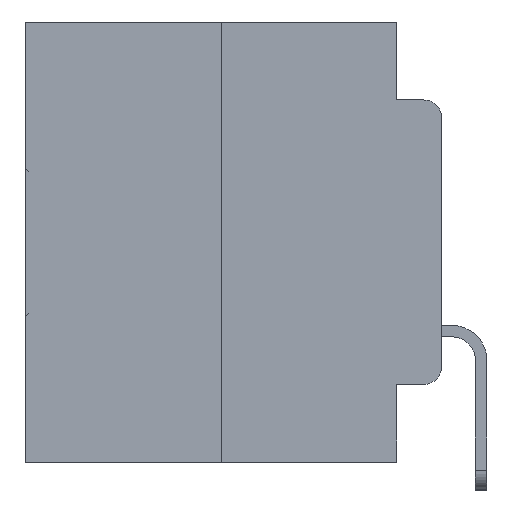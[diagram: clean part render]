
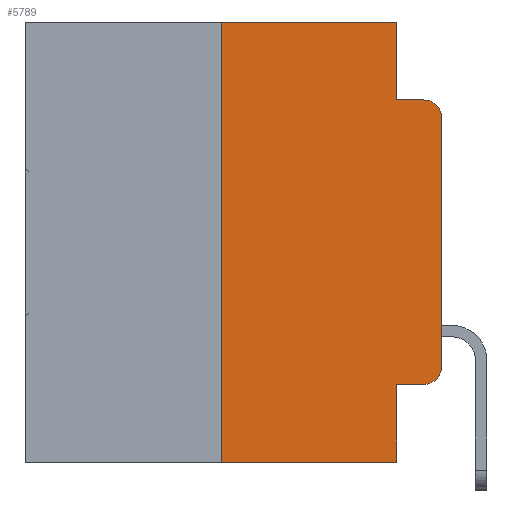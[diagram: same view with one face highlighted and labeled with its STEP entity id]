
A CAD part, left-side view. The second image highlights one B-rep face of the part: STEP entity #5789.
In plain terms, the highlighted planar face has unit normal (-1, 0, 0).
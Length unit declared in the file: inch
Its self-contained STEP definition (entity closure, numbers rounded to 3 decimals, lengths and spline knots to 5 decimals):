
#359 = VERTEX_POINT ( 'NONE', #4496 ) ;
#924 = VERTEX_POINT ( 'NONE', #22224 ) ;
#1751 = LINE ( 'NONE', #13528, #19166 ) ;
#1945 = LINE ( 'NONE', #23768, #21489 ) ;
#2202 = VERTEX_POINT ( 'NONE', #22669 ) ;
#2836 = CARTESIAN_POINT ( 'NONE',  ( 0., 0.051, 0. ) ) ;
#3096 = VERTEX_POINT ( 'NONE', #24365 ) ;
#3116 = PLANE ( 'NONE',  #24971 ) ;
#3329 = DIRECTION ( 'NONE',  ( 0., 0., -1. ) ) ;
#4472 = VECTOR ( 'NONE', #3329, 39.37008 ) ;
#4486 = CARTESIAN_POINT ( 'NONE',  ( 0., 0.02, -0.1085 ) ) ;
#4496 = CARTESIAN_POINT ( 'NONE',  ( 0., 0.051, -0.0885 ) ) ;
#4574 = DIRECTION ( 'NONE',  ( 0., 0., -1. ) ) ;
#4781 = CARTESIAN_POINT ( 'NONE',  ( 0., 0., 0. ) ) ;
#4948 = DIRECTION ( 'NONE',  ( -1., 0., 0. ) ) ;
#5156 = VERTEX_POINT ( 'NONE', #26609 ) ;
#5623 = CIRCLE ( 'NONE', #19106, 0.02 ) ;
#5789 = ADVANCED_FACE ( 'NONE', ( #25299 ), #3116, .F. ) ;
#6085 = LINE ( 'NONE', #24752, #14557 ) ;
#7357 = VECTOR ( 'NONE', #22712, 39.37008 ) ;
#7671 = EDGE_CURVE ( 'NONE', #359, #26872, #6085, .T. ) ;
#7709 = CARTESIAN_POINT ( 'NONE',  ( 0., 0.051, 0. ) ) ;
#7758 = LINE ( 'NONE', #12530, #8471 ) ;
#7809 = AXIS2_PLACEMENT_3D ( 'NONE', #18550, #4948, #20825 ) ;
#7986 = ORIENTED_EDGE ( 'NONE', *, *, #7671, .F. ) ;
#8322 = EDGE_CURVE ( 'NONE', #11139, #23448, #1751, .T. ) ;
#8471 = VECTOR ( 'NONE', #23954, 39.37008 ) ;
#8658 = EDGE_CURVE ( 'NONE', #20943, #26930, #7758, .T. ) ;
#8813 = DIRECTION ( 'NONE',  ( 0., -1., 0. ) ) ;
#9169 = EDGE_CURVE ( 'NONE', #20943, #11139, #15193, .T. ) ;
#10482 = EDGE_CURVE ( 'NONE', #3096, #924, #17296, .T. ) ;
#11045 = VECTOR ( 'NONE', #11236, 39.37008 ) ;
#11139 = VERTEX_POINT ( 'NONE', #11206 ) ;
#11167 = EDGE_CURVE ( 'NONE', #924, #26872, #5623, .T. ) ;
#11206 = CARTESIAN_POINT ( 'NONE',  ( 0., 0.25, 0. ) ) ;
#11236 = DIRECTION ( 'NONE',  ( 0., 0., -1. ) ) ;
#11402 = ORIENTED_EDGE ( 'NONE', *, *, #8322, .F. ) ;
#11656 = VECTOR ( 'NONE', #15746, 39.37008 ) ;
#12154 = ORIENTED_EDGE ( 'NONE', *, *, #26990, .T. ) ;
#12530 = CARTESIAN_POINT ( 'NONE',  ( 0., 0.473, -0.5 ) ) ;
#12810 = ORIENTED_EDGE ( 'NONE', *, *, #9169, .F. ) ;
#12998 = ORIENTED_EDGE ( 'NONE', *, *, #10482, .T. ) ;
#13528 = CARTESIAN_POINT ( 'NONE',  ( 0., 0.473, 0. ) ) ;
#14422 = CARTESIAN_POINT ( 'NONE',  ( 0., 0.051, -0.5 ) ) ;
#14557 = VECTOR ( 'NONE', #8813, 39.37008 ) ;
#14722 = CARTESIAN_POINT ( 'NONE',  ( 0., 0.02, -0.0885 ) ) ;
#15089 = DIRECTION ( 'NONE',  ( 0., 0., -1. ) ) ;
#15157 = EDGE_CURVE ( 'NONE', #5156, #26930, #21157, .T. ) ;
#15193 = LINE ( 'NONE', #27140, #11656 ) ;
#15746 = DIRECTION ( 'NONE',  ( 0., 0., 1. ) ) ;
#16046 = EDGE_CURVE ( 'NONE', #2202, #3096, #25396, .T. ) ;
#17296 = LINE ( 'NONE', #4781, #7357 ) ;
#17542 = ORIENTED_EDGE ( 'NONE', *, *, #22540, .F. ) ;
#18465 = DIRECTION ( 'NONE',  ( -1., 0., 0. ) ) ;
#18550 = CARTESIAN_POINT ( 'NONE',  ( 0., 0.02, -0.3915 ) ) ;
#18883 = ORIENTED_EDGE ( 'NONE', *, *, #16046, .T. ) ;
#19106 = AXIS2_PLACEMENT_3D ( 'NONE', #4486, #18465, #4574 ) ;
#19166 = VECTOR ( 'NONE', #20363, 39.37008 ) ;
#20363 = DIRECTION ( 'NONE',  ( 0., -1., 0. ) ) ;
#20825 = DIRECTION ( 'NONE',  ( 0., 0., -1. ) ) ;
#20943 = VERTEX_POINT ( 'NONE', #24436 ) ;
#21157 = LINE ( 'NONE', #2836, #4472 ) ;
#21489 = VECTOR ( 'NONE', #28393, 39.37008 ) ;
#21700 = LINE ( 'NONE', #27077, #11045 ) ;
#21736 = CARTESIAN_POINT ( 'NONE',  ( 0., 0.473, 0. ) ) ;
#22224 = CARTESIAN_POINT ( 'NONE',  ( 0., 0., -0.1085 ) ) ;
#22329 = ORIENTED_EDGE ( 'NONE', *, *, #15157, .F. ) ;
#22540 = EDGE_CURVE ( 'NONE', #23448, #359, #21700, .T. ) ;
#22669 = CARTESIAN_POINT ( 'NONE',  ( 0., 0.02, -0.4115 ) ) ;
#22712 = DIRECTION ( 'NONE',  ( 0., 0., 1. ) ) ;
#23448 = VERTEX_POINT ( 'NONE', #7709 ) ;
#23576 = ORIENTED_EDGE ( 'NONE', *, *, #8658, .T. ) ;
#23768 = CARTESIAN_POINT ( 'NONE',  ( 0., 0.051, -0.4115 ) ) ;
#23954 = DIRECTION ( 'NONE',  ( 0., -1., 0. ) ) ;
#24365 = CARTESIAN_POINT ( 'NONE',  ( 0., 0., -0.3915 ) ) ;
#24436 = CARTESIAN_POINT ( 'NONE',  ( 0., 0.25, -0.5 ) ) ;
#24752 = CARTESIAN_POINT ( 'NONE',  ( 0., 0.051, -0.0885 ) ) ;
#24971 = AXIS2_PLACEMENT_3D ( 'NONE', #21736, #28461, #15089 ) ;
#25299 = FACE_OUTER_BOUND ( 'NONE', #28462, .T. ) ;
#25396 = CIRCLE ( 'NONE', #7809, 0.02 ) ;
#26609 = CARTESIAN_POINT ( 'NONE',  ( 0., 0.051, -0.4115 ) ) ;
#26872 = VERTEX_POINT ( 'NONE', #14722 ) ;
#26930 = VERTEX_POINT ( 'NONE', #14422 ) ;
#26990 = EDGE_CURVE ( 'NONE', #5156, #2202, #1945, .T. ) ;
#27077 = CARTESIAN_POINT ( 'NONE',  ( 0., 0.051, 0. ) ) ;
#27140 = CARTESIAN_POINT ( 'NONE',  ( 0., 0.25, 0. ) ) ;
#28393 = DIRECTION ( 'NONE',  ( 0., -1., 0. ) ) ;
#28461 = DIRECTION ( 'NONE',  ( 1., 0., 0. ) ) ;
#28462 = EDGE_LOOP ( 'NONE', ( #12998, #29123, #7986, #17542, #11402, #12810, #23576, #22329, #12154, #18883 ) ) ;
#29123 = ORIENTED_EDGE ( 'NONE', *, *, #11167, .T. ) ;
